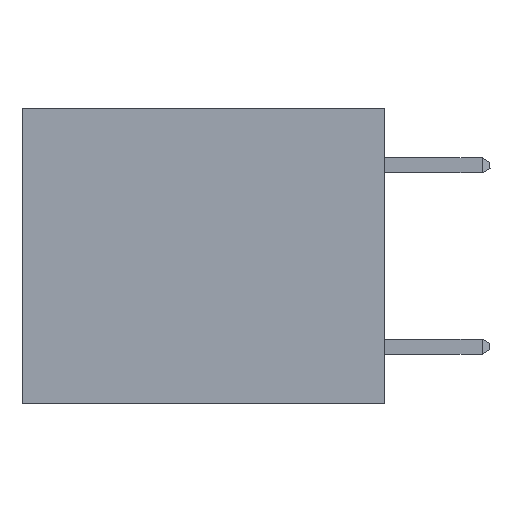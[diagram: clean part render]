
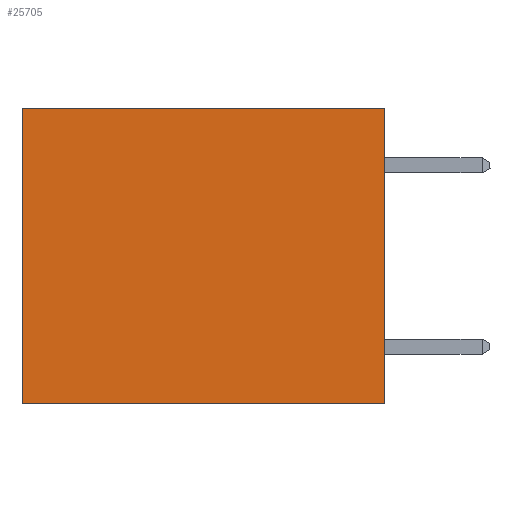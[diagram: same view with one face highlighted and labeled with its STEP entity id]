
A CAD part, left-side view. The second image highlights one B-rep face of the part: STEP entity #25705.
In plain terms, the highlighted planar face has unit normal (-1, 0, 0).
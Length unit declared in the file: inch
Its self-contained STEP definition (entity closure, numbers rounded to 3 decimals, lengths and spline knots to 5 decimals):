
#1768 = EDGE_CURVE ( 'NONE', #22879, #17286, #11710, .T. ) ;
#2114 = LINE ( 'NONE', #25053, #27183 ) ;
#2757 = FACE_OUTER_BOUND ( 'NONE', #27826, .T. ) ;
#3055 = EDGE_CURVE ( 'NONE', #19359, #16952, #2114, .T. ) ;
#3240 = ORIENTED_EDGE ( 'NONE', *, *, #1768, .T. ) ;
#5716 = DIRECTION ( 'NONE',  ( 0., 1., 0. ) ) ;
#6589 = CARTESIAN_POINT ( 'NONE',  ( 0.3165, 0.6, -0.49 ) ) ;
#9499 = VECTOR ( 'NONE', #30402, 39.37008 ) ;
#10264 = LINE ( 'NONE', #6589, #9499 ) ;
#11002 = DIRECTION ( 'NONE',  ( 0., 1., 0. ) ) ;
#11343 = DIRECTION ( 'NONE',  ( 1., 0., 0. ) ) ;
#11545 = PLANE ( 'NONE',  #22518 ) ;
#11710 = LINE ( 'NONE', #20192, #20053 ) ;
#12141 = EDGE_CURVE ( 'NONE', #22879, #19359, #24246, .T. ) ;
#13915 = VECTOR ( 'NONE', #23484, 39.37008 ) ;
#14492 = CARTESIAN_POINT ( 'NONE',  ( 0.3165, 0.6, -0.49 ) ) ;
#15474 = ORIENTED_EDGE ( 'NONE', *, *, #27570, .T. ) ;
#16522 = CARTESIAN_POINT ( 'NONE',  ( 0.3165, 0., -0.49 ) ) ;
#16952 = VERTEX_POINT ( 'NONE', #14492 ) ;
#17286 = VERTEX_POINT ( 'NONE', #19623 ) ;
#18588 = CARTESIAN_POINT ( 'NONE',  ( 0.3165, 0., -0.49 ) ) ;
#18847 = CARTESIAN_POINT ( 'NONE',  ( 0.3165, 0., -0.49 ) ) ;
#19359 = VERTEX_POINT ( 'NONE', #18847 ) ;
#19623 = CARTESIAN_POINT ( 'NONE',  ( 0.3165, 0.6, 0. ) ) ;
#20053 = VECTOR ( 'NONE', #5716, 39.37008 ) ;
#20192 = CARTESIAN_POINT ( 'NONE',  ( 0.3165, 0., 0. ) ) ;
#22518 = AXIS2_PLACEMENT_3D ( 'NONE', #16522, #11343, #23890 ) ;
#22879 = VERTEX_POINT ( 'NONE', #27096 ) ;
#23204 = ORIENTED_EDGE ( 'NONE', *, *, #3055, .F. ) ;
#23484 = DIRECTION ( 'NONE',  ( 0., 0., -1. ) ) ;
#23890 = DIRECTION ( 'NONE',  ( 0., 0., -1. ) ) ;
#24246 = LINE ( 'NONE', #18588, #13915 ) ;
#25053 = CARTESIAN_POINT ( 'NONE',  ( 0.3165, 0., -0.49 ) ) ;
#25121 = ORIENTED_EDGE ( 'NONE', *, *, #12141, .F. ) ;
#25705 = ADVANCED_FACE ( 'NONE', ( #2757 ), #11545, .F. ) ;
#27096 = CARTESIAN_POINT ( 'NONE',  ( 0.3165, 0., 0. ) ) ;
#27183 = VECTOR ( 'NONE', #11002, 39.37008 ) ;
#27570 = EDGE_CURVE ( 'NONE', #17286, #16952, #10264, .T. ) ;
#27826 = EDGE_LOOP ( 'NONE', ( #15474, #23204, #25121, #3240 ) ) ;
#30402 = DIRECTION ( 'NONE',  ( 0., 0., -1. ) ) ;
